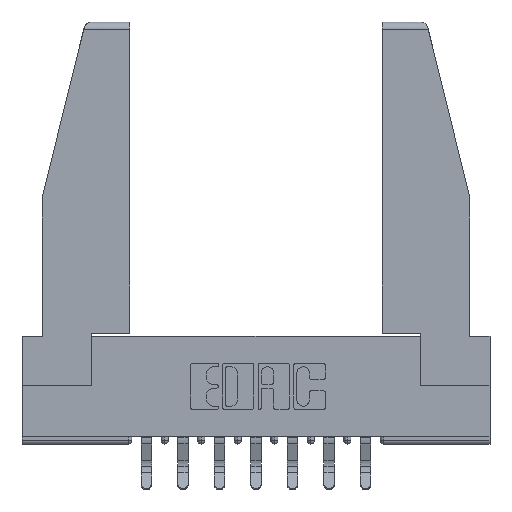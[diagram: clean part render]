
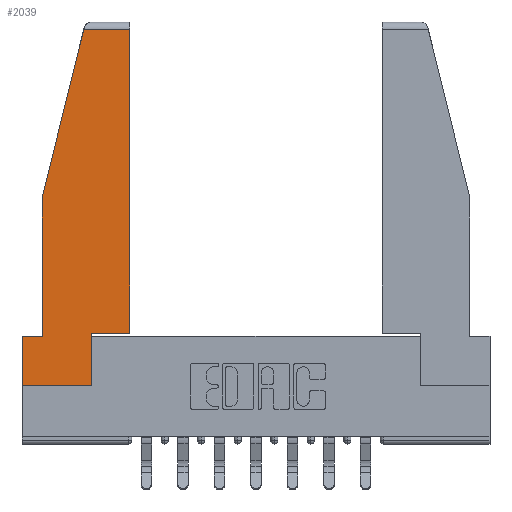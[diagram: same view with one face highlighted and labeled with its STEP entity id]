
A CAD part, top view. The second image highlights one B-rep face of the part: STEP entity #2039.
In plain terms, the highlighted planar face has unit normal (0, 0, 1).
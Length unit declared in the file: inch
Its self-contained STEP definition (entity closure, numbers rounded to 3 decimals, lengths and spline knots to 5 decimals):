
#1001 = VECTOR ( 'NONE', #3674, 39.37008 ) ;
#1591 = CARTESIAN_POINT ( 'NONE',  ( 0., 1.52, 0. ) ) ;
#1597 = ORIENTED_EDGE ( 'NONE', *, *, #5357, .T. ) ;
#1887 = VERTEX_POINT ( 'NONE', #6616 ) ;
#2039 = ADVANCED_FACE ( 'NONE', ( #3973 ), #4638, .T. ) ;
#2602 = LINE ( 'NONE', #5018, #7311 ) ;
#2801 = VERTEX_POINT ( 'NONE', #7858 ) ;
#3320 = VERTEX_POINT ( 'NONE', #6784 ) ;
#3482 = CARTESIAN_POINT ( 'NONE',  ( 0.297, 0., 0. ) ) ;
#3539 = CARTESIAN_POINT ( 'NONE',  ( 0.297, 0.223, 0. ) ) ;
#3674 = DIRECTION ( 'NONE',  ( -1., 0., 0. ) ) ;
#3973 = FACE_OUTER_BOUND ( 'NONE', #6656, .T. ) ;
#4110 = LINE ( 'NONE', #12400, #4824 ) ;
#4259 = ORIENTED_EDGE ( 'NONE', *, *, #6272, .T. ) ;
#4279 = LINE ( 'NONE', #3539, #11812 ) ;
#4396 = EDGE_CURVE ( 'NONE', #5420, #12079, #12393, .T. ) ;
#4409 = CARTESIAN_POINT ( 'NONE',  ( 0.297, 0.223, 0. ) ) ;
#4593 = DIRECTION ( 'NONE',  ( 1., 0., 0. ) ) ;
#4622 = VECTOR ( 'NONE', #8782, 39.37008 ) ;
#4638 = PLANE ( 'NONE',  #7347 ) ;
#4824 = VECTOR ( 'NONE', #6677, 39.37008 ) ;
#5018 = CARTESIAN_POINT ( 'NONE',  ( 0.271, 1.55, 0. ) ) ;
#5357 = EDGE_CURVE ( 'NONE', #1887, #5420, #5385, .T. ) ;
#5385 = LINE ( 'NONE', #6984, #8143 ) ;
#5388 = VECTOR ( 'NONE', #8960, 39.37008 ) ;
#5420 = VERTEX_POINT ( 'NONE', #10267 ) ;
#5572 = CARTESIAN_POINT ( 'NONE',  ( 0.086, 0.8, 0. ) ) ;
#5918 = VERTEX_POINT ( 'NONE', #5572 ) ;
#6272 = EDGE_CURVE ( 'NONE', #3320, #12621, #4110, .T. ) ;
#6591 = DIRECTION ( 'NONE',  ( -1., 0., 0. ) ) ;
#6616 = CARTESIAN_POINT ( 'NONE',  ( 0.461, 0.223, 0. ) ) ;
#6656 = EDGE_LOOP ( 'NONE', ( #1597, #12536, #11658, #10518, #10997, #4259, #14478, #8477, #9096 ) ) ;
#6677 = DIRECTION ( 'NONE',  ( 0., -1., 0. ) ) ;
#6784 = CARTESIAN_POINT ( 'NONE',  ( 0., 0.21, 0. ) ) ;
#6984 = CARTESIAN_POINT ( 'NONE',  ( 0.461, 0.223, 0. ) ) ;
#7014 = LINE ( 'NONE', #8594, #8409 ) ;
#7132 = EDGE_CURVE ( 'NONE', #2801, #3320, #13145, .T. ) ;
#7143 = DIRECTION ( 'NONE',  ( -0.239, -0.971, 0. ) ) ;
#7311 = VECTOR ( 'NONE', #7143, 39.37008 ) ;
#7347 = AXIS2_PLACEMENT_3D ( 'NONE', #10153, #13477, #4593 ) ;
#7397 = VECTOR ( 'NONE', #6591, 39.37008 ) ;
#7760 = EDGE_CURVE ( 'NONE', #12621, #13044, #8628, .T. ) ;
#7781 = DIRECTION ( 'NONE',  ( 1., 0., 0. ) ) ;
#7858 = CARTESIAN_POINT ( 'NONE',  ( 0.086, 0.21, 0. ) ) ;
#8143 = VECTOR ( 'NONE', #11349, 39.37008 ) ;
#8409 = VECTOR ( 'NONE', #9669, 39.37008 ) ;
#8477 = ORIENTED_EDGE ( 'NONE', *, *, #10957, .T. ) ;
#8594 = CARTESIAN_POINT ( 'NONE',  ( 0.086, 0.8, 0. ) ) ;
#8628 = LINE ( 'NONE', #12338, #4622 ) ;
#8782 = DIRECTION ( 'NONE',  ( 1., 0., 0. ) ) ;
#8791 = EDGE_CURVE ( 'NONE', #5918, #2801, #7014, .T. ) ;
#8868 = CARTESIAN_POINT ( 'NONE',  ( 0.2636, 1.52, 0. ) ) ;
#8960 = DIRECTION ( 'NONE',  ( 0., 1., 0. ) ) ;
#9096 = ORIENTED_EDGE ( 'NONE', *, *, #12709, .T. ) ;
#9669 = DIRECTION ( 'NONE',  ( 0., -1., 0. ) ) ;
#10153 = CARTESIAN_POINT ( 'NONE',  ( 0., 0., 0. ) ) ;
#10267 = CARTESIAN_POINT ( 'NONE',  ( 0.461, 1.52, 0. ) ) ;
#10502 = EDGE_CURVE ( 'NONE', #12079, #5918, #2602, .T. ) ;
#10518 = ORIENTED_EDGE ( 'NONE', *, *, #8791, .T. ) ;
#10957 = EDGE_CURVE ( 'NONE', #13044, #12612, #14289, .T. ) ;
#10997 = ORIENTED_EDGE ( 'NONE', *, *, #7132, .T. ) ;
#11349 = DIRECTION ( 'NONE',  ( 0., 1., 0. ) ) ;
#11658 = ORIENTED_EDGE ( 'NONE', *, *, #10502, .T. ) ;
#11812 = VECTOR ( 'NONE', #7781, 39.37008 ) ;
#12079 = VERTEX_POINT ( 'NONE', #8868 ) ;
#12338 = CARTESIAN_POINT ( 'NONE',  ( 0., 0., 0. ) ) ;
#12393 = LINE ( 'NONE', #1591, #1001 ) ;
#12400 = CARTESIAN_POINT ( 'NONE',  ( 0., 0.21, 0. ) ) ;
#12536 = ORIENTED_EDGE ( 'NONE', *, *, #4396, .T. ) ;
#12612 = VERTEX_POINT ( 'NONE', #4409 ) ;
#12621 = VERTEX_POINT ( 'NONE', #14532 ) ;
#12709 = EDGE_CURVE ( 'NONE', #12612, #1887, #4279, .T. ) ;
#13044 = VERTEX_POINT ( 'NONE', #13212 ) ;
#13145 = LINE ( 'NONE', #13284, #7397 ) ;
#13212 = CARTESIAN_POINT ( 'NONE',  ( 0.297, 0., 0. ) ) ;
#13284 = CARTESIAN_POINT ( 'NONE',  ( 0., 0.21, 0. ) ) ;
#13477 = DIRECTION ( 'NONE',  ( 0., 0., 1. ) ) ;
#14289 = LINE ( 'NONE', #3482, #5388 ) ;
#14478 = ORIENTED_EDGE ( 'NONE', *, *, #7760, .T. ) ;
#14532 = CARTESIAN_POINT ( 'NONE',  ( 0., 0., 0. ) ) ;
